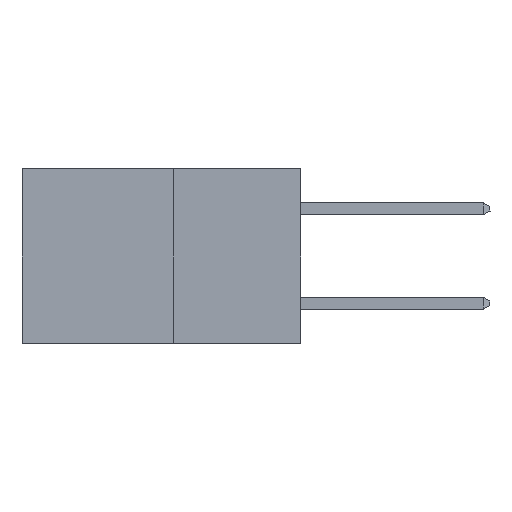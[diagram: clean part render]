
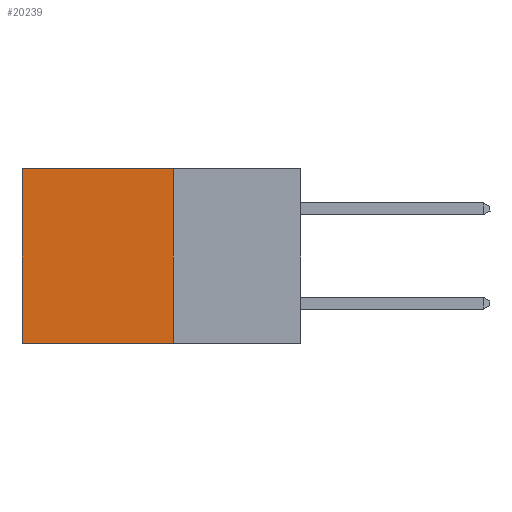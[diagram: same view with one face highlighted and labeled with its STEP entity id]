
A CAD part, left-side view. The second image highlights one B-rep face of the part: STEP entity #20239.
In plain terms, the highlighted planar face has unit normal (-1, 0, 0).
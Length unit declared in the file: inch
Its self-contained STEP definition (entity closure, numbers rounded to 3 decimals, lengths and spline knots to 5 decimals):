
#1699 = VERTEX_POINT ( 'NONE', #8462 ) ;
#2740 = LINE ( 'NONE', #15974, #3354 ) ;
#3152 = LINE ( 'NONE', #5057, #23841 ) ;
#3354 = VECTOR ( 'NONE', #17886, 39.37008 ) ;
#4654 = DIRECTION ( 'NONE',  ( 0., 1., 0. ) ) ;
#5044 = ORIENTED_EDGE ( 'NONE', *, *, #16812, .T. ) ;
#5057 = CARTESIAN_POINT ( 'NONE',  ( 0.277, 0.59, -0.37 ) ) ;
#5129 = DIRECTION ( 'NONE',  ( 0., 0., -1. ) ) ;
#5561 = EDGE_LOOP ( 'NONE', ( #6775, #6396, #16337, #5044 ) ) ;
#6205 = LINE ( 'NONE', #11736, #11301 ) ;
#6396 = ORIENTED_EDGE ( 'NONE', *, *, #9584, .F. ) ;
#6775 = ORIENTED_EDGE ( 'NONE', *, *, #7895, .T. ) ;
#7406 = PLANE ( 'NONE',  #23981 ) ;
#7895 = EDGE_CURVE ( 'NONE', #1699, #9933, #3152, .T. ) ;
#8462 = CARTESIAN_POINT ( 'NONE',  ( 0.277, 0.59, 0. ) ) ;
#9327 = DIRECTION ( 'NONE',  ( 1., 0., 0. ) ) ;
#9584 = EDGE_CURVE ( 'NONE', #16209, #9933, #12383, .T. ) ;
#9933 = VERTEX_POINT ( 'NONE', #11463 ) ;
#11301 = VECTOR ( 'NONE', #21139, 39.37008 ) ;
#11428 = VERTEX_POINT ( 'NONE', #21306 ) ;
#11463 = CARTESIAN_POINT ( 'NONE',  ( 0.277, 0.59, -0.37 ) ) ;
#11736 = CARTESIAN_POINT ( 'NONE',  ( 0.277, 0.27, -0.37 ) ) ;
#12383 = LINE ( 'NONE', #21775, #22943 ) ;
#14223 = CARTESIAN_POINT ( 'NONE',  ( 0.277, 0.27, -0.37 ) ) ;
#15974 = CARTESIAN_POINT ( 'NONE',  ( 0.277, 0.27, 0. ) ) ;
#16209 = VERTEX_POINT ( 'NONE', #14223 ) ;
#16337 = ORIENTED_EDGE ( 'NONE', *, *, #22220, .F. ) ;
#16812 = EDGE_CURVE ( 'NONE', #11428, #1699, #2740, .T. ) ;
#17886 = DIRECTION ( 'NONE',  ( 0., 1., 0. ) ) ;
#20239 = ADVANCED_FACE ( 'NONE', ( #22515 ), #7406, .F. ) ;
#20639 = CARTESIAN_POINT ( 'NONE',  ( 0.277, 0.27, -0.37 ) ) ;
#21139 = DIRECTION ( 'NONE',  ( 0., 0., -1. ) ) ;
#21306 = CARTESIAN_POINT ( 'NONE',  ( 0.277, 0.27, 0. ) ) ;
#21775 = CARTESIAN_POINT ( 'NONE',  ( 0.277, 0.27, -0.37 ) ) ;
#22220 = EDGE_CURVE ( 'NONE', #11428, #16209, #6205, .T. ) ;
#22473 = DIRECTION ( 'NONE',  ( 0., 0., -1. ) ) ;
#22515 = FACE_OUTER_BOUND ( 'NONE', #5561, .T. ) ;
#22943 = VECTOR ( 'NONE', #4654, 39.37008 ) ;
#23841 = VECTOR ( 'NONE', #5129, 39.37008 ) ;
#23981 = AXIS2_PLACEMENT_3D ( 'NONE', #20639, #9327, #22473 ) ;
